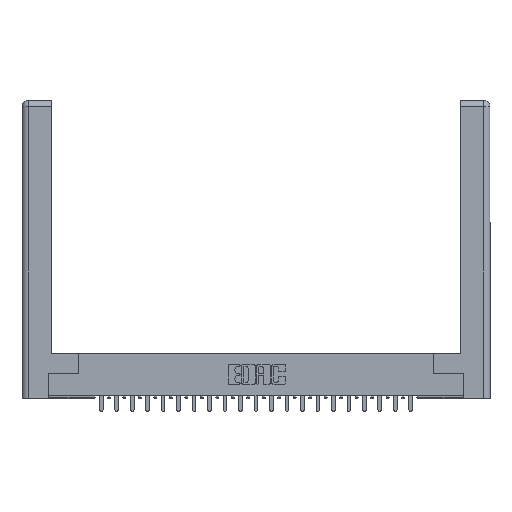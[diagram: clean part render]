
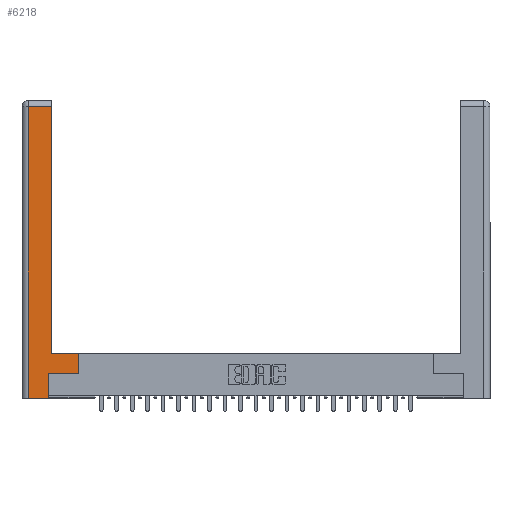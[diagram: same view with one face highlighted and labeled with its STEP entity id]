
A CAD part, top view. The second image highlights one B-rep face of the part: STEP entity #6218.
In plain terms, the highlighted planar face has unit normal (0, 0, 1).
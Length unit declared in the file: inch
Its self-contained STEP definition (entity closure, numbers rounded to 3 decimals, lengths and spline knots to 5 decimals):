
#38 = LINE ( 'NONE', #23105, #1168 ) ;
#915 = VERTEX_POINT ( 'NONE', #9720 ) ;
#998 = DIRECTION ( 'NONE',  ( 1., 0., 0. ) ) ;
#1048 = ORIENTED_EDGE ( 'NONE', *, *, #7499, .T. ) ;
#1168 = VECTOR ( 'NONE', #1686, 39.37008 ) ;
#1207 = CARTESIAN_POINT ( 'NONE',  ( 0.295, 0.45, 0. ) ) ;
#1254 = VERTEX_POINT ( 'NONE', #7688 ) ;
#1686 = DIRECTION ( 'NONE',  ( 1., 0., 0. ) ) ;
#2140 = CARTESIAN_POINT ( 'NONE',  ( 0.265, 0.245, 0. ) ) ;
#2349 = AXIS2_PLACEMENT_3D ( 'NONE', #23139, #5749, #9512 ) ;
#2389 = ORIENTED_EDGE ( 'NONE', *, *, #9548, .T. ) ;
#3263 = CARTESIAN_POINT ( 'NONE',  ( 0.0615, 2.94, 0. ) ) ;
#3346 = DIRECTION ( 'NONE',  ( 0., 1., 0. ) ) ;
#3427 = DIRECTION ( 'NONE',  ( -1., 0., 0. ) ) ;
#3593 = CARTESIAN_POINT ( 'NONE',  ( 0.565, 0.45, 0. ) ) ;
#4073 = EDGE_CURVE ( 'NONE', #12800, #17256, #14762, .T. ) ;
#4652 = LINE ( 'NONE', #14370, #5267 ) ;
#4938 = VERTEX_POINT ( 'NONE', #1207 ) ;
#5267 = VECTOR ( 'NONE', #998, 39.37008 ) ;
#5444 = EDGE_CURVE ( 'NONE', #17256, #915, #19781, .T. ) ;
#5470 = DIRECTION ( 'NONE',  ( 0., 1., 0. ) ) ;
#5635 = EDGE_CURVE ( 'NONE', #915, #18431, #4652, .T. ) ;
#5662 = VECTOR ( 'NONE', #3346, 39.37008 ) ;
#5749 = DIRECTION ( 'NONE',  ( 0., 0., -1. ) ) ;
#6082 = EDGE_CURVE ( 'NONE', #6679, #4938, #6390, .T. ) ;
#6218 = ADVANCED_FACE ( 'NONE', ( #23391 ), #21106, .F. ) ;
#6274 = LINE ( 'NONE', #2140, #12481 ) ;
#6390 = LINE ( 'NONE', #16467, #24838 ) ;
#6461 = ORIENTED_EDGE ( 'NONE', *, *, #5635, .T. ) ;
#6529 = EDGE_CURVE ( 'NONE', #1254, #6679, #14804, .T. ) ;
#6679 = VERTEX_POINT ( 'NONE', #9877 ) ;
#7499 = EDGE_CURVE ( 'NONE', #18431, #9061, #6274, .T. ) ;
#7612 = CARTESIAN_POINT ( 'NONE',  ( 0.0615, 0., 0. ) ) ;
#7636 = EDGE_LOOP ( 'NONE', ( #2389, #20364, #14376, #6461, #1048, #24521, #18701, #17500 ) ) ;
#7688 = CARTESIAN_POINT ( 'NONE',  ( 0.565, 0.245, 0. ) ) ;
#7748 = CARTESIAN_POINT ( 'NONE',  ( 0.295, 3., 0. ) ) ;
#8051 = DIRECTION ( 'NONE',  ( 0., 1., 0. ) ) ;
#9061 = VERTEX_POINT ( 'NONE', #13565 ) ;
#9512 = DIRECTION ( 'NONE',  ( -1., 0., 0. ) ) ;
#9548 = EDGE_CURVE ( 'NONE', #4938, #12800, #18827, .T. ) ;
#9720 = CARTESIAN_POINT ( 'NONE',  ( 0.0615, 0., 0. ) ) ;
#9877 = CARTESIAN_POINT ( 'NONE',  ( 0.565, 0.45, 0. ) ) ;
#10856 = CARTESIAN_POINT ( 'NONE',  ( 0.265, 0., 0. ) ) ;
#12481 = VECTOR ( 'NONE', #8051, 39.37008 ) ;
#12800 = VERTEX_POINT ( 'NONE', #24150 ) ;
#13565 = CARTESIAN_POINT ( 'NONE',  ( 0.265, 0.245, 0. ) ) ;
#14094 = DIRECTION ( 'NONE',  ( -1., 0., 0. ) ) ;
#14370 = CARTESIAN_POINT ( 'NONE',  ( 0.265, 0., 0. ) ) ;
#14376 = ORIENTED_EDGE ( 'NONE', *, *, #5444, .T. ) ;
#14762 = LINE ( 'NONE', #21044, #21237 ) ;
#14804 = LINE ( 'NONE', #3593, #5662 ) ;
#16467 = CARTESIAN_POINT ( 'NONE',  ( 0.295, 0.45, 0. ) ) ;
#17256 = VERTEX_POINT ( 'NONE', #3263 ) ;
#17500 = ORIENTED_EDGE ( 'NONE', *, *, #6082, .T. ) ;
#18166 = EDGE_CURVE ( 'NONE', #9061, #1254, #38, .T. ) ;
#18431 = VERTEX_POINT ( 'NONE', #10856 ) ;
#18701 = ORIENTED_EDGE ( 'NONE', *, *, #6529, .T. ) ;
#18827 = LINE ( 'NONE', #7748, #19812 ) ;
#19071 = DIRECTION ( 'NONE',  ( 0., -1., 0. ) ) ;
#19337 = VECTOR ( 'NONE', #19071, 39.37008 ) ;
#19781 = LINE ( 'NONE', #7612, #19337 ) ;
#19812 = VECTOR ( 'NONE', #5470, 39.37008 ) ;
#20364 = ORIENTED_EDGE ( 'NONE', *, *, #4073, .T. ) ;
#21044 = CARTESIAN_POINT ( 'NONE',  ( 0.0615, 2.94, 0. ) ) ;
#21106 = PLANE ( 'NONE',  #2349 ) ;
#21237 = VECTOR ( 'NONE', #3427, 39.37008 ) ;
#23105 = CARTESIAN_POINT ( 'NONE',  ( 0.565, 0.245, 0. ) ) ;
#23139 = CARTESIAN_POINT ( 'NONE',  ( 0., 0., 0. ) ) ;
#23391 = FACE_OUTER_BOUND ( 'NONE', #7636, .T. ) ;
#24150 = CARTESIAN_POINT ( 'NONE',  ( 0.295, 2.94, 0. ) ) ;
#24521 = ORIENTED_EDGE ( 'NONE', *, *, #18166, .T. ) ;
#24838 = VECTOR ( 'NONE', #14094, 39.37008 ) ;
